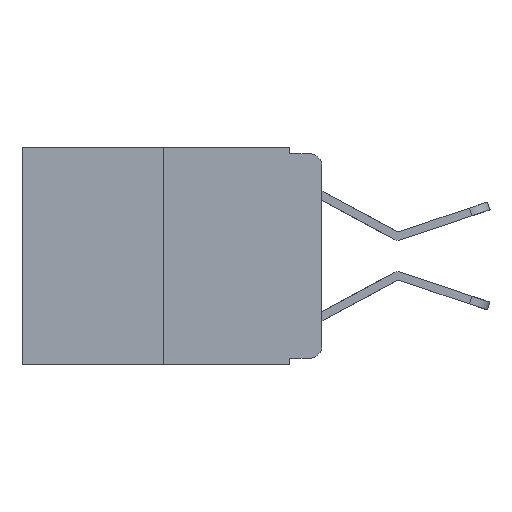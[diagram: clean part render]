
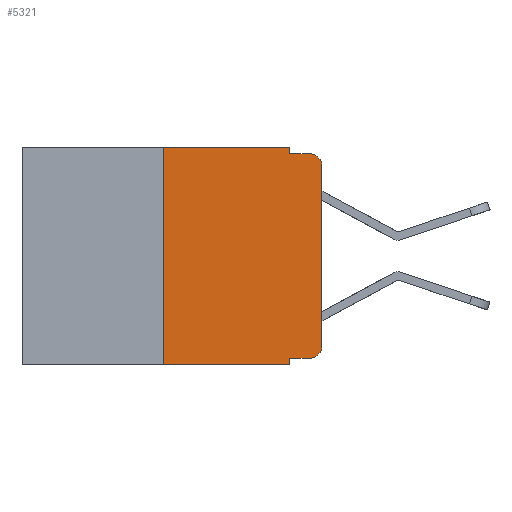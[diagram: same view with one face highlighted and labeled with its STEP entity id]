
A CAD part, left-side view. The second image highlights one B-rep face of the part: STEP entity #5321.
In plain terms, the highlighted planar face has unit normal (-1, 0, 0).
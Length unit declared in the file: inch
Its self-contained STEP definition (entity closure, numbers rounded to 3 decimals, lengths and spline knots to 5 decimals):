
#391 = AXIS2_PLACEMENT_3D ( 'NONE', #409, #11809, #11884 ) ;
#409 = CARTESIAN_POINT ( 'NONE',  ( 0., 0.02, -0.03 ) ) ;
#411 = ORIENTED_EDGE ( 'NONE', *, *, #1266, .F. ) ;
#674 = VERTEX_POINT ( 'NONE', #7394 ) ;
#710 = LINE ( 'NONE', #13152, #10331 ) ;
#1004 = AXIS2_PLACEMENT_3D ( 'NONE', #7807, #10931, #10841 ) ;
#1047 = DIRECTION ( 'NONE',  ( 0., 0., -1. ) ) ;
#1150 = VECTOR ( 'NONE', #5109, 39.37008 ) ;
#1266 = EDGE_CURVE ( 'NONE', #3846, #674, #14300, .T. ) ;
#1313 = DIRECTION ( 'NONE',  ( 0., 0., -1. ) ) ;
#1678 = ORIENTED_EDGE ( 'NONE', *, *, #2052, .T. ) ;
#1770 = AXIS2_PLACEMENT_3D ( 'NONE', #7401, #8977, #13258 ) ;
#2052 = EDGE_CURVE ( 'NONE', #2355, #10912, #6129, .T. ) ;
#2303 = EDGE_CURVE ( 'NONE', #11104, #11390, #5487, .T. ) ;
#2336 = ORIENTED_EDGE ( 'NONE', *, *, #2622, .F. ) ;
#2355 = VERTEX_POINT ( 'NONE', #13723 ) ;
#2612 = VECTOR ( 'NONE', #13070, 39.37008 ) ;
#2622 = EDGE_CURVE ( 'NONE', #674, #6322, #710, .T. ) ;
#2879 = EDGE_CURVE ( 'NONE', #10912, #15971, #13562, .T. ) ;
#3134 = EDGE_CURVE ( 'NONE', #6322, #15971, #9522, .T. ) ;
#3139 = DIRECTION ( 'NONE',  ( 0., 0., 1. ) ) ;
#3142 = CARTESIAN_POINT ( 'NONE',  ( 0., 0.02, -0.01 ) ) ;
#3619 = CARTESIAN_POINT ( 'NONE',  ( 0., 0.051, -0.01 ) ) ;
#3846 = VERTEX_POINT ( 'NONE', #7097 ) ;
#3898 = LINE ( 'NONE', #12841, #1150 ) ;
#3916 = EDGE_CURVE ( 'NONE', #10710, #2355, #7290, .T. ) ;
#4008 = VECTOR ( 'NONE', #8146, 39.37008 ) ;
#4015 = ORIENTED_EDGE ( 'NONE', *, *, #11734, .F. ) ;
#5092 = CARTESIAN_POINT ( 'NONE',  ( 0., 0.051, -0.333 ) ) ;
#5109 = DIRECTION ( 'NONE',  ( 0., -1., 0. ) ) ;
#5201 = FACE_OUTER_BOUND ( 'NONE', #16503, .T. ) ;
#5321 = ADVANCED_FACE ( 'NONE', ( #5201 ), #10855, .F. ) ;
#5487 = LINE ( 'NONE', #8162, #15304 ) ;
#5859 = CARTESIAN_POINT ( 'NONE',  ( 0., 0.25, -0.343 ) ) ;
#6070 = ORIENTED_EDGE ( 'NONE', *, *, #2879, .T. ) ;
#6129 = LINE ( 'NONE', #15677, #16647 ) ;
#6322 = VERTEX_POINT ( 'NONE', #3619 ) ;
#6415 = DIRECTION ( 'NONE',  ( 0., -1., 0. ) ) ;
#7097 = CARTESIAN_POINT ( 'NONE',  ( 0., 0.25, 0. ) ) ;
#7290 = CIRCLE ( 'NONE', #1770, 0.02 ) ;
#7394 = CARTESIAN_POINT ( 'NONE',  ( 0., 0.051, 0. ) ) ;
#7401 = CARTESIAN_POINT ( 'NONE',  ( 0., 0.02, -0.313 ) ) ;
#7404 = EDGE_CURVE ( 'NONE', #8035, #10710, #3898, .T. ) ;
#7807 = CARTESIAN_POINT ( 'NONE',  ( 0., 0.473, 0. ) ) ;
#8035 = VERTEX_POINT ( 'NONE', #5092 ) ;
#8146 = DIRECTION ( 'NONE',  ( 0., -1., 0. ) ) ;
#8162 = CARTESIAN_POINT ( 'NONE',  ( 0., 0.473, -0.343 ) ) ;
#8908 = CARTESIAN_POINT ( 'NONE',  ( 0., 0.051, 0. ) ) ;
#8977 = DIRECTION ( 'NONE',  ( -1., 0., 0. ) ) ;
#9283 = CARTESIAN_POINT ( 'NONE',  ( 0., 0., -0.03 ) ) ;
#9522 = LINE ( 'NONE', #11843, #2612 ) ;
#9894 = ORIENTED_EDGE ( 'NONE', *, *, #3916, .T. ) ;
#9980 = EDGE_CURVE ( 'NONE', #8035, #11390, #15794, .T. ) ;
#10268 = ORIENTED_EDGE ( 'NONE', *, *, #3134, .F. ) ;
#10331 = VECTOR ( 'NONE', #1313, 39.37008 ) ;
#10710 = VERTEX_POINT ( 'NONE', #12847 ) ;
#10841 = DIRECTION ( 'NONE',  ( 0., 0., -1. ) ) ;
#10855 = PLANE ( 'NONE',  #1004 ) ;
#10912 = VERTEX_POINT ( 'NONE', #9283 ) ;
#10931 = DIRECTION ( 'NONE',  ( 1., 0., 0. ) ) ;
#11104 = VERTEX_POINT ( 'NONE', #5859 ) ;
#11390 = VERTEX_POINT ( 'NONE', #16514 ) ;
#11734 = EDGE_CURVE ( 'NONE', #11104, #3846, #15173, .T. ) ;
#11809 = DIRECTION ( 'NONE',  ( -1., 0., 0. ) ) ;
#11823 = VECTOR ( 'NONE', #3139, 39.37008 ) ;
#11843 = CARTESIAN_POINT ( 'NONE',  ( 0., 0.051, -0.01 ) ) ;
#11884 = DIRECTION ( 'NONE',  ( 0., 0., -1. ) ) ;
#12841 = CARTESIAN_POINT ( 'NONE',  ( 0., 0.051, -0.333 ) ) ;
#12847 = CARTESIAN_POINT ( 'NONE',  ( 0., 0.02, -0.333 ) ) ;
#12935 = ORIENTED_EDGE ( 'NONE', *, *, #7404, .T. ) ;
#13070 = DIRECTION ( 'NONE',  ( 0., -1., 0. ) ) ;
#13152 = CARTESIAN_POINT ( 'NONE',  ( 0., 0.051, 0. ) ) ;
#13258 = DIRECTION ( 'NONE',  ( 0., 0., -1. ) ) ;
#13562 = CIRCLE ( 'NONE', #391, 0.02 ) ;
#13723 = CARTESIAN_POINT ( 'NONE',  ( 0., 0., -0.313 ) ) ;
#14300 = LINE ( 'NONE', #14312, #4008 ) ;
#14312 = CARTESIAN_POINT ( 'NONE',  ( 0., 0.473, 0. ) ) ;
#15173 = LINE ( 'NONE', #15912, #11823 ) ;
#15304 = VECTOR ( 'NONE', #6415, 39.37008 ) ;
#15459 = ORIENTED_EDGE ( 'NONE', *, *, #2303, .T. ) ;
#15677 = CARTESIAN_POINT ( 'NONE',  ( 0., 0., 0. ) ) ;
#15748 = DIRECTION ( 'NONE',  ( 0., 0., 1. ) ) ;
#15794 = LINE ( 'NONE', #8908, #16186 ) ;
#15828 = ORIENTED_EDGE ( 'NONE', *, *, #9980, .F. ) ;
#15912 = CARTESIAN_POINT ( 'NONE',  ( 0., 0.25, 0. ) ) ;
#15971 = VERTEX_POINT ( 'NONE', #3142 ) ;
#16186 = VECTOR ( 'NONE', #1047, 39.37008 ) ;
#16503 = EDGE_LOOP ( 'NONE', ( #1678, #6070, #10268, #2336, #411, #4015, #15459, #15828, #12935, #9894 ) ) ;
#16514 = CARTESIAN_POINT ( 'NONE',  ( 0., 0.051, -0.343 ) ) ;
#16647 = VECTOR ( 'NONE', #15748, 39.37008 ) ;
